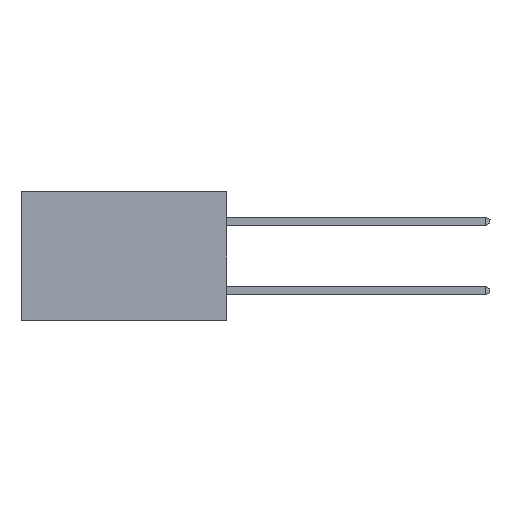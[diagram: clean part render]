
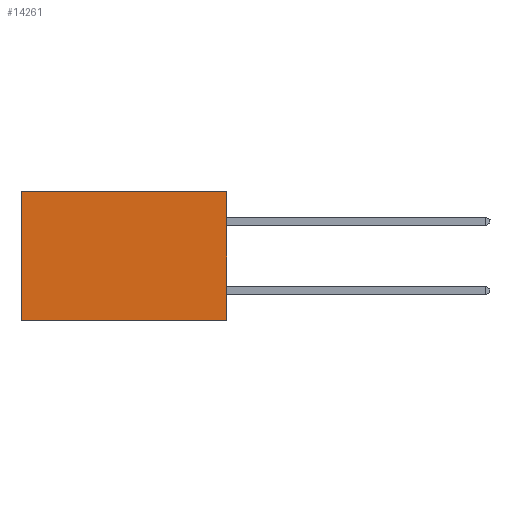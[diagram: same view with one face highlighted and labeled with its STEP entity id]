
A CAD part, left-side view. The second image highlights one B-rep face of the part: STEP entity #14261.
In plain terms, the highlighted planar face has unit normal (-1, 0, 0).
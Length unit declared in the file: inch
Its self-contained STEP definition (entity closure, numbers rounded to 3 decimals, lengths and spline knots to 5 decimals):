
#851 = EDGE_CURVE ( 'NONE', #7562, #14402, #3966, .T. ) ;
#867 = VECTOR ( 'NONE', #10801, 39.37008 ) ;
#1246 = EDGE_CURVE ( 'NONE', #13247, #15156, #9714, .T. ) ;
#2434 = CARTESIAN_POINT ( 'NONE',  ( 0.277, 0., 0. ) ) ;
#2591 = EDGE_CURVE ( 'NONE', #14402, #15156, #5535, .T. ) ;
#2962 = CARTESIAN_POINT ( 'NONE',  ( 0.277, 0., -0.37 ) ) ;
#3350 = CARTESIAN_POINT ( 'NONE',  ( 0.277, 0., -0.37 ) ) ;
#3966 = LINE ( 'NONE', #20480, #21883 ) ;
#4741 = DIRECTION ( 'NONE',  ( 1., 0., 0. ) ) ;
#5535 = LINE ( 'NONE', #7142, #14257 ) ;
#7125 = DIRECTION ( 'NONE',  ( 0., 1., 0. ) ) ;
#7142 = CARTESIAN_POINT ( 'NONE',  ( 0.277, 0., -0.37 ) ) ;
#7562 = VERTEX_POINT ( 'NONE', #2434 ) ;
#8192 = AXIS2_PLACEMENT_3D ( 'NONE', #2962, #4741, #16915 ) ;
#8502 = EDGE_LOOP ( 'NONE', ( #21028, #11950, #18314, #16980 ) ) ;
#9714 = LINE ( 'NONE', #12467, #867 ) ;
#10276 = DIRECTION ( 'NONE',  ( 0., 0., -1. ) ) ;
#10554 = CARTESIAN_POINT ( 'NONE',  ( 0.277, 0.59, -0.37 ) ) ;
#10801 = DIRECTION ( 'NONE',  ( 0., 0., -1. ) ) ;
#11950 = ORIENTED_EDGE ( 'NONE', *, *, #2591, .F. ) ;
#12467 = CARTESIAN_POINT ( 'NONE',  ( 0.277, 0.59, -0.37 ) ) ;
#13247 = VERTEX_POINT ( 'NONE', #18983 ) ;
#13440 = PLANE ( 'NONE',  #8192 ) ;
#13568 = DIRECTION ( 'NONE',  ( 0., 1., 0. ) ) ;
#14257 = VECTOR ( 'NONE', #7125, 39.37008 ) ;
#14261 = ADVANCED_FACE ( 'NONE', ( #21873 ), #13440, .F. ) ;
#14402 = VERTEX_POINT ( 'NONE', #3350 ) ;
#14986 = EDGE_CURVE ( 'NONE', #7562, #13247, #20802, .T. ) ;
#15156 = VERTEX_POINT ( 'NONE', #10554 ) ;
#16915 = DIRECTION ( 'NONE',  ( 0., 0., -1. ) ) ;
#16980 = ORIENTED_EDGE ( 'NONE', *, *, #14986, .T. ) ;
#18314 = ORIENTED_EDGE ( 'NONE', *, *, #851, .F. ) ;
#18619 = CARTESIAN_POINT ( 'NONE',  ( 0.277, 0., 0. ) ) ;
#18983 = CARTESIAN_POINT ( 'NONE',  ( 0.277, 0.59, 0. ) ) ;
#20258 = VECTOR ( 'NONE', #13568, 39.37008 ) ;
#20480 = CARTESIAN_POINT ( 'NONE',  ( 0.277, 0., -0.37 ) ) ;
#20802 = LINE ( 'NONE', #18619, #20258 ) ;
#21028 = ORIENTED_EDGE ( 'NONE', *, *, #1246, .T. ) ;
#21873 = FACE_OUTER_BOUND ( 'NONE', #8502, .T. ) ;
#21883 = VECTOR ( 'NONE', #10276, 39.37008 ) ;
